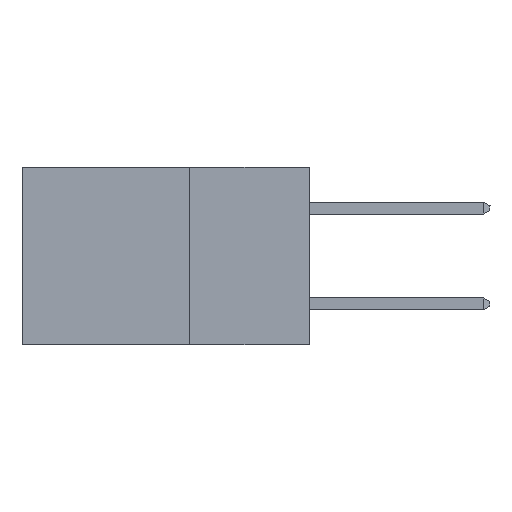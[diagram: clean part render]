
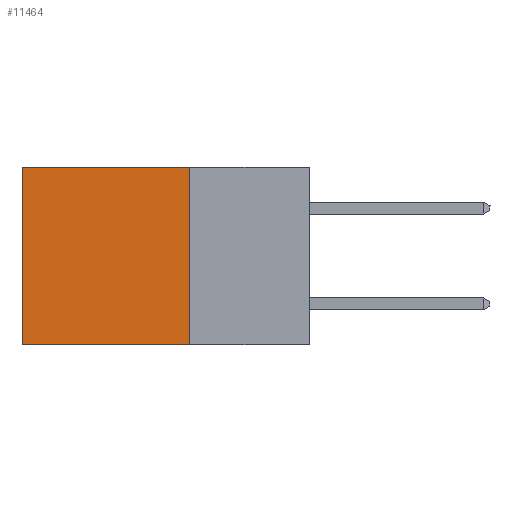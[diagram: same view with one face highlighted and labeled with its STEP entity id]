
A CAD part, left-side view. The second image highlights one B-rep face of the part: STEP entity #11464.
In plain terms, the highlighted planar face has unit normal (-1, 0, 0).
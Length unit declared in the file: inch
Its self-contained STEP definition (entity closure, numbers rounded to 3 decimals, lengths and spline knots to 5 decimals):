
#183 = DIRECTION ( 'NONE',  ( 0., 1., 0. ) ) ;
#1404 = LINE ( 'NONE', #28917, #10037 ) ;
#3418 = FACE_OUTER_BOUND ( 'NONE', #31339, .T. ) ;
#3476 = CARTESIAN_POINT ( 'NONE',  ( 0.2875, 0.6, -0.37 ) ) ;
#4763 = ORIENTED_EDGE ( 'NONE', *, *, #39274, .T. ) ;
#5448 = VERTEX_POINT ( 'NONE', #41941 ) ;
#6529 = VERTEX_POINT ( 'NONE', #26148 ) ;
#6662 = LINE ( 'NONE', #27332, #25767 ) ;
#9393 = VECTOR ( 'NONE', #22506, 39.37008 ) ;
#9473 = ORIENTED_EDGE ( 'NONE', *, *, #39593, .T. ) ;
#10037 = VECTOR ( 'NONE', #183, 39.37008 ) ;
#10550 = LINE ( 'NONE', #11920, #9393 ) ;
#11464 = ADVANCED_FACE ( 'NONE', ( #3418 ), #13367, .F. ) ;
#11920 = CARTESIAN_POINT ( 'NONE',  ( 0.2875, 0.25, -0.37 ) ) ;
#12736 = ORIENTED_EDGE ( 'NONE', *, *, #40223, .F. ) ;
#13367 = PLANE ( 'NONE',  #29229 ) ;
#13553 = EDGE_CURVE ( 'NONE', #37913, #6529, #35610, .T. ) ;
#17012 = DIRECTION ( 'NONE',  ( 1., 0., 0. ) ) ;
#22506 = DIRECTION ( 'NONE',  ( 0., 1., 0. ) ) ;
#23957 = CARTESIAN_POINT ( 'NONE',  ( 0.2875, 0.25, 0. ) ) ;
#25767 = VECTOR ( 'NONE', #30576, 39.37008 ) ;
#26148 = CARTESIAN_POINT ( 'NONE',  ( 0.2875, 0.25, -0.37 ) ) ;
#27332 = CARTESIAN_POINT ( 'NONE',  ( 0.2875, 0.6, 0. ) ) ;
#28917 = CARTESIAN_POINT ( 'NONE',  ( 0.2875, 0.25, 0. ) ) ;
#29229 = AXIS2_PLACEMENT_3D ( 'NONE', #23957, #17012, #41056 ) ;
#29784 = CARTESIAN_POINT ( 'NONE',  ( 0.2875, 0.25, 0. ) ) ;
#30244 = DIRECTION ( 'NONE',  ( 0., 0., -1. ) ) ;
#30576 = DIRECTION ( 'NONE',  ( 0., 0., -1. ) ) ;
#31339 = EDGE_LOOP ( 'NONE', ( #4763, #12736, #42388, #9473 ) ) ;
#33426 = CARTESIAN_POINT ( 'NONE',  ( 0.2875, 0.25, 0. ) ) ;
#35355 = VECTOR ( 'NONE', #30244, 39.37008 ) ;
#35610 = LINE ( 'NONE', #33426, #35355 ) ;
#37913 = VERTEX_POINT ( 'NONE', #29784 ) ;
#39274 = EDGE_CURVE ( 'NONE', #5448, #45302, #6662, .T. ) ;
#39593 = EDGE_CURVE ( 'NONE', #37913, #5448, #1404, .T. ) ;
#40223 = EDGE_CURVE ( 'NONE', #6529, #45302, #10550, .T. ) ;
#41056 = DIRECTION ( 'NONE',  ( 0., 0., -1. ) ) ;
#41941 = CARTESIAN_POINT ( 'NONE',  ( 0.2875, 0.6, 0. ) ) ;
#42388 = ORIENTED_EDGE ( 'NONE', *, *, #13553, .F. ) ;
#45302 = VERTEX_POINT ( 'NONE', #3476 ) ;
